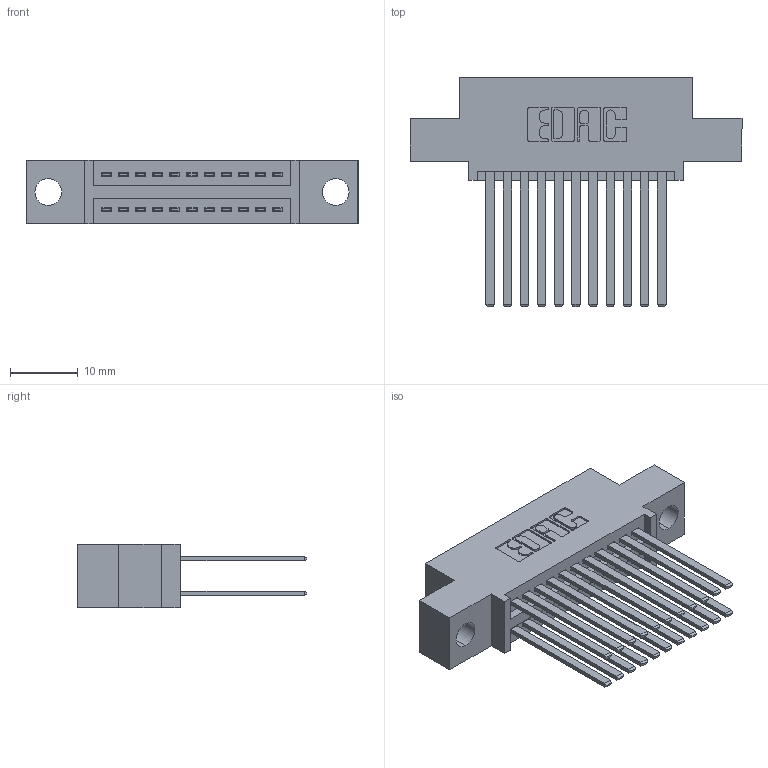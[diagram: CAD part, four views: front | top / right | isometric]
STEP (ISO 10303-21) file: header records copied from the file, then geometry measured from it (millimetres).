
FILE_DESCRIPTION (( 'STEP AP203' ), '1' );
FILE_NAME ('345-022-544-504.STEP', '2021-05-19T22:11:39', ( '' ), ( '' ), 'SwSTEP 2.0', 'SolidWorks 2020', '' );
FILE_SCHEMA (( 'CONFIG_CONTROL_DESIGN' ));
Length unit declared in the file: inch
Products named in the file (3): 345 Part_0.110 Offset - 0.156 Dia-TI; 345-022-544-504; 345-292-001_345-293-144
Assembly tree (23 placements, depth 2):
  345-022-544-504
    345 Part_0.110 Offset - 0.156 Dia-TI
    345-292-001_345-293-144  x22
Bounding box: 49.15 x 33.96 x 9.4 mm (x, y, z)
Volume: 4615.7 mm3; surface area: 7070.7 mm2
Topology: 23 solids, 23 shells, 1112 faces, 3271 edges, 2150 vertices
Faces by surface type: plane 736, cylinder 376
Entity records: 13171 total; most frequent: CARTESIAN_POINT 2242, ORIENTED_EDGE 2174, DIRECTION 2011, EDGE_CURVE 1087, LINE 915, VECTOR 915, VERTEX_POINT 722, AXIS2_PLACEMENT_3D 548
